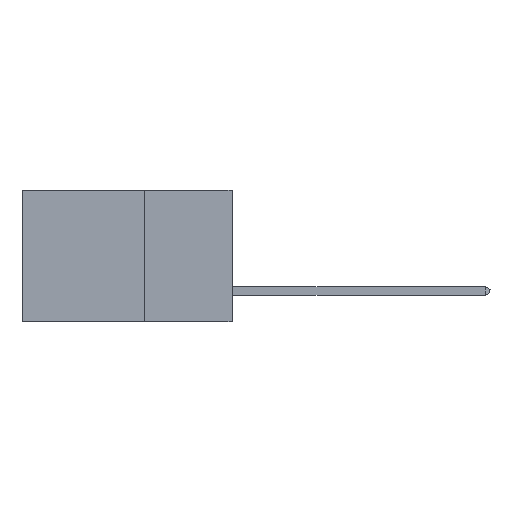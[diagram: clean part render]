
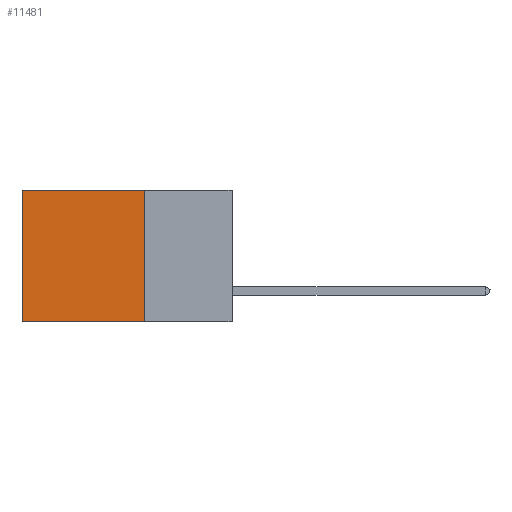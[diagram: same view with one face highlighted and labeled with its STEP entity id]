
A CAD part, left-side view. The second image highlights one B-rep face of the part: STEP entity #11481.
In plain terms, the highlighted planar face has unit normal (-1, 0, 0).
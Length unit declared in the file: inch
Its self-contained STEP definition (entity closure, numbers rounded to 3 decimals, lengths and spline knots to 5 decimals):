
#481 = CARTESIAN_POINT ( 'NONE',  ( 0.2875, 0.6, -0.375 ) ) ;
#553 = LINE ( 'NONE', #4745, #8668 ) ;
#1130 = EDGE_CURVE ( 'NONE', #10243, #12881, #8458, .T. ) ;
#1678 = DIRECTION ( 'NONE',  ( 1., 0., 0. ) ) ;
#1764 = ORIENTED_EDGE ( 'NONE', *, *, #12506, .T. ) ;
#1897 = ORIENTED_EDGE ( 'NONE', *, *, #11465, .F. ) ;
#2282 = VECTOR ( 'NONE', #6552, 39.37008 ) ;
#2283 = VERTEX_POINT ( 'NONE', #12261 ) ;
#2419 = EDGE_LOOP ( 'NONE', ( #1764, #11873, #1897, #11154 ) ) ;
#2465 = CARTESIAN_POINT ( 'NONE',  ( 0.2875, 0.25, 0. ) ) ;
#4004 = CARTESIAN_POINT ( 'NONE',  ( 0.2875, 0.25, -0.375 ) ) ;
#4164 = VECTOR ( 'NONE', #6547, 39.37008 ) ;
#4745 = CARTESIAN_POINT ( 'NONE',  ( 0.2875, 0.25, -0.375 ) ) ;
#4814 = CARTESIAN_POINT ( 'NONE',  ( 0.2875, 0.6, -0.375 ) ) ;
#4828 = AXIS2_PLACEMENT_3D ( 'NONE', #8833, #1678, #9773 ) ;
#5242 = VERTEX_POINT ( 'NONE', #9913 ) ;
#5505 = CARTESIAN_POINT ( 'NONE',  ( 0.2875, 0.25, -0.375 ) ) ;
#5679 = FACE_OUTER_BOUND ( 'NONE', #2419, .T. ) ;
#6547 = DIRECTION ( 'NONE',  ( 0., 1., 0. ) ) ;
#6552 = DIRECTION ( 'NONE',  ( 0., 0., -1. ) ) ;
#7570 = DIRECTION ( 'NONE',  ( 0., 1., 0. ) ) ;
#7748 = LINE ( 'NONE', #2465, #4164 ) ;
#8458 = LINE ( 'NONE', #5505, #12480 ) ;
#8668 = VECTOR ( 'NONE', #12756, 39.37008 ) ;
#8768 = LINE ( 'NONE', #4814, #2282 ) ;
#8833 = CARTESIAN_POINT ( 'NONE',  ( 0.2875, 0.25, -0.375 ) ) ;
#9773 = DIRECTION ( 'NONE',  ( 0., 0., -1. ) ) ;
#9913 = CARTESIAN_POINT ( 'NONE',  ( 0.2875, 0.6, 0. ) ) ;
#10165 = EDGE_CURVE ( 'NONE', #2283, #5242, #7748, .T. ) ;
#10243 = VERTEX_POINT ( 'NONE', #4004 ) ;
#11154 = ORIENTED_EDGE ( 'NONE', *, *, #10165, .T. ) ;
#11465 = EDGE_CURVE ( 'NONE', #2283, #10243, #553, .T. ) ;
#11481 = ADVANCED_FACE ( 'NONE', ( #5679 ), #11623, .F. ) ;
#11623 = PLANE ( 'NONE',  #4828 ) ;
#11873 = ORIENTED_EDGE ( 'NONE', *, *, #1130, .F. ) ;
#12261 = CARTESIAN_POINT ( 'NONE',  ( 0.2875, 0.25, 0. ) ) ;
#12480 = VECTOR ( 'NONE', #7570, 39.37008 ) ;
#12506 = EDGE_CURVE ( 'NONE', #5242, #12881, #8768, .T. ) ;
#12756 = DIRECTION ( 'NONE',  ( 0., 0., -1. ) ) ;
#12881 = VERTEX_POINT ( 'NONE', #481 ) ;
